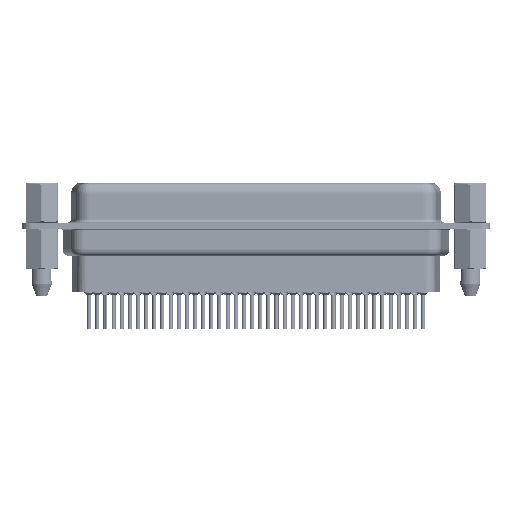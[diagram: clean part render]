
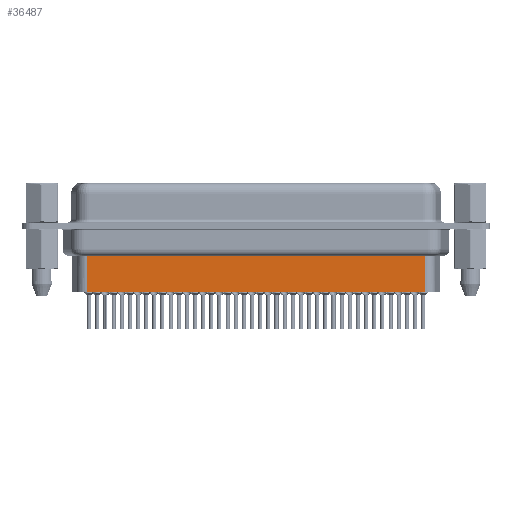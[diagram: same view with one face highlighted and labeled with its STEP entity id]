
A CAD part, front view. The second image highlights one B-rep face of the part: STEP entity #36487.
In plain terms, the highlighted planar face has unit normal (0, -1, 0).
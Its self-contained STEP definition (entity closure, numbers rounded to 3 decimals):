
#1681 = DIRECTION ( 'NONE',  ( -1., 0., 0. ) ) ;
#4302 = EDGE_CURVE ( 'NONE', #48731, #42284, #23901, .T. ) ;
#5113 = CARTESIAN_POINT ( 'NONE',  ( 56.794, -3.5, -9.85 ) ) ;
#5901 = CARTESIAN_POINT ( 'NONE',  ( 56.794, -3.5, -4.097 ) ) ;
#6572 = LINE ( 'NONE', #51278, #41941 ) ;
#7649 = EDGE_LOOP ( 'NONE', ( #42767, #33123, #36597, #22460 ) ) ;
#8438 = VECTOR ( 'NONE', #46587, 1000. ) ;
#8852 = DIRECTION ( 'NONE',  ( 1., 0., 0. ) ) ;
#10762 = CARTESIAN_POINT ( 'NONE',  ( 6.459, -3.5, -4.097 ) ) ;
#15667 = DIRECTION ( 'NONE',  ( 0., 0., -1. ) ) ;
#16463 = CARTESIAN_POINT ( 'NONE',  ( 6.706, -3.5, -4.097 ) ) ;
#16612 = CARTESIAN_POINT ( 'NONE',  ( 6.706, -3.5, -3.1 ) ) ;
#18248 = LINE ( 'NONE', #10762, #28297 ) ;
#20061 = FACE_OUTER_BOUND ( 'NONE', #7649, .T. ) ;
#20603 = PLANE ( 'NONE',  #36993 ) ;
#22255 = CARTESIAN_POINT ( 'NONE',  ( 56.794, -3.5, -3.1 ) ) ;
#22460 = ORIENTED_EDGE ( 'NONE', *, *, #4302, .F. ) ;
#22903 = VERTEX_POINT ( 'NONE', #16463 ) ;
#23901 = LINE ( 'NONE', #39680, #28002 ) ;
#28002 = VECTOR ( 'NONE', #39956, 1000. ) ;
#28297 = VECTOR ( 'NONE', #1681, 1000. ) ;
#30599 = EDGE_CURVE ( 'NONE', #42790, #48731, #46869, .T. ) ;
#32891 = DIRECTION ( 'NONE',  ( 0., -1., 0. ) ) ;
#33123 = ORIENTED_EDGE ( 'NONE', *, *, #45268, .T. ) ;
#34486 = EDGE_CURVE ( 'NONE', #22903, #42284, #6572, .T. ) ;
#36487 = ADVANCED_FACE ( 'NONE', ( #20061 ), #20603, .T. ) ;
#36597 = ORIENTED_EDGE ( 'NONE', *, *, #34486, .T. ) ;
#36993 = AXIS2_PLACEMENT_3D ( 'NONE', #16612, #32891, #8852 ) ;
#39680 = CARTESIAN_POINT ( 'NONE',  ( 6.706, -3.5, -9.85 ) ) ;
#39956 = DIRECTION ( 'NONE',  ( -1., 0., 0. ) ) ;
#41941 = VECTOR ( 'NONE', #15667, 1000. ) ;
#42284 = VERTEX_POINT ( 'NONE', #43527 ) ;
#42767 = ORIENTED_EDGE ( 'NONE', *, *, #30599, .F. ) ;
#42790 = VERTEX_POINT ( 'NONE', #5901 ) ;
#43527 = CARTESIAN_POINT ( 'NONE',  ( 6.706, -3.5, -9.85 ) ) ;
#45268 = EDGE_CURVE ( 'NONE', #42790, #22903, #18248, .T. ) ;
#46587 = DIRECTION ( 'NONE',  ( 0., 0., -1. ) ) ;
#46869 = LINE ( 'NONE', #22255, #8438 ) ;
#48731 = VERTEX_POINT ( 'NONE', #5113 ) ;
#51278 = CARTESIAN_POINT ( 'NONE',  ( 6.706, -3.5, -3.1 ) ) ;
